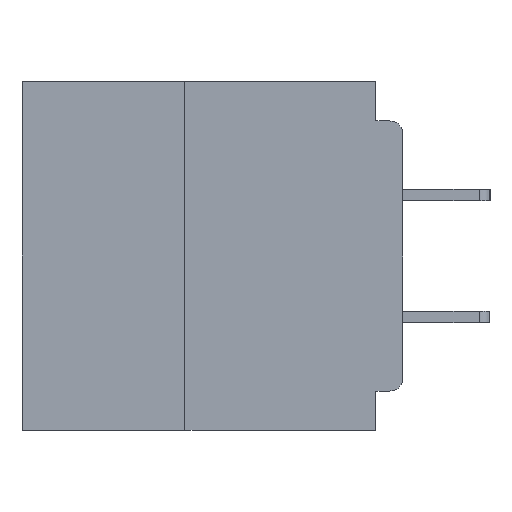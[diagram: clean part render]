
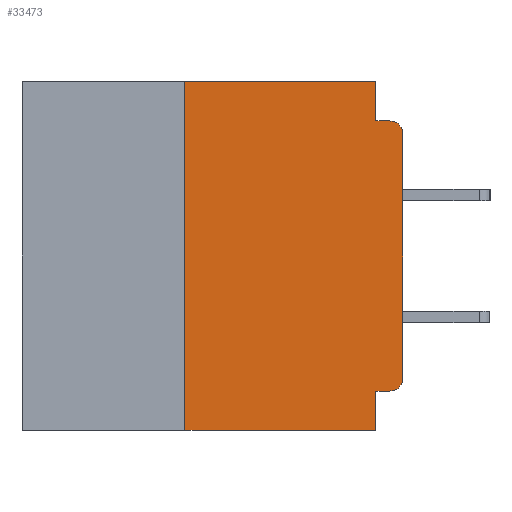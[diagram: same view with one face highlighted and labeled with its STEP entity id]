
A CAD part, left-side view. The second image highlights one B-rep face of the part: STEP entity #33473.
In plain terms, the highlighted planar face has unit normal (-1, 0, 0).
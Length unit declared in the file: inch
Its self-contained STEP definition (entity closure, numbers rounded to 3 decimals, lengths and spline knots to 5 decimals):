
#336 = LINE ( 'NONE', #9048, #36361 ) ;
#529 = LINE ( 'NONE', #7827, #14073 ) ;
#898 = EDGE_CURVE ( 'NONE', #4974, #16801, #36397, .T. ) ;
#1073 = EDGE_CURVE ( 'NONE', #11123, #27617, #28911, .T. ) ;
#1193 = EDGE_CURVE ( 'NONE', #33816, #10783, #336, .T. ) ;
#1250 = EDGE_CURVE ( 'NONE', #16801, #27617, #6198, .T. ) ;
#1259 = CARTESIAN_POINT ( 'NONE',  ( 0., 0.031, 0. ) ) ;
#1301 = EDGE_CURVE ( 'NONE', #33816, #4974, #20012, .T. ) ;
#1632 = ORIENTED_EDGE ( 'NONE', *, *, #10062, .T. ) ;
#2718 = CARTESIAN_POINT ( 'NONE',  ( 0., 0.031, -0.4 ) ) ;
#4177 = VECTOR ( 'NONE', #7340, 39.37008 ) ;
#4974 = VERTEX_POINT ( 'NONE', #30198 ) ;
#5546 = ORIENTED_EDGE ( 'NONE', *, *, #9873, .F. ) ;
#6198 = CIRCLE ( 'NONE', #20914, 0.015 ) ;
#7340 = DIRECTION ( 'NONE',  ( 0., 0., -1. ) ) ;
#7827 = CARTESIAN_POINT ( 'NONE',  ( 0., 0.25, -0.4 ) ) ;
#8604 = VECTOR ( 'NONE', #20373, 39.37008 ) ;
#9048 = CARTESIAN_POINT ( 'NONE',  ( 0., 0., -0.355 ) ) ;
#9590 = CARTESIAN_POINT ( 'NONE',  ( 0., 0., -0.045 ) ) ;
#9873 = EDGE_CURVE ( 'NONE', #22394, #11123, #27360, .T. ) ;
#9991 = EDGE_CURVE ( 'NONE', #13685, #15500, #529, .T. ) ;
#10062 = EDGE_CURVE ( 'NONE', #13685, #33516, #19256, .T. ) ;
#10125 = EDGE_CURVE ( 'NONE', #10783, #33516, #16416, .T. ) ;
#10783 = VERTEX_POINT ( 'NONE', #28747 ) ;
#11123 = VERTEX_POINT ( 'NONE', #24500 ) ;
#12314 = ORIENTED_EDGE ( 'NONE', *, *, #898, .T. ) ;
#13685 = VERTEX_POINT ( 'NONE', #15130 ) ;
#13720 = CARTESIAN_POINT ( 'NONE',  ( 0., 0.437, 0. ) ) ;
#13733 = CARTESIAN_POINT ( 'NONE',  ( 0., 0., 0. ) ) ;
#13835 = CARTESIAN_POINT ( 'NONE',  ( 0., 0.015, -0.355 ) ) ;
#14073 = VECTOR ( 'NONE', #16563, 39.37008 ) ;
#14253 = DIRECTION ( 'NONE',  ( 0., 1., 0. ) ) ;
#14795 = CARTESIAN_POINT ( 'NONE',  ( 0., 0.015, -0.045 ) ) ;
#15130 = CARTESIAN_POINT ( 'NONE',  ( 0., 0.25, -0.4 ) ) ;
#15298 = DIRECTION ( 'NONE',  ( 1., 0., 0. ) ) ;
#15500 = VERTEX_POINT ( 'NONE', #15547 ) ;
#15547 = CARTESIAN_POINT ( 'NONE',  ( 0., 0.25, 0. ) ) ;
#16416 = LINE ( 'NONE', #2718, #8604 ) ;
#16563 = DIRECTION ( 'NONE',  ( 0., 0., 1. ) ) ;
#16748 = CARTESIAN_POINT ( 'NONE',  ( 0., 0., -0.06 ) ) ;
#16801 = VERTEX_POINT ( 'NONE', #16748 ) ;
#16952 = CARTESIAN_POINT ( 'NONE',  ( 0., 0.437, -0.4 ) ) ;
#17098 = ORIENTED_EDGE ( 'NONE', *, *, #10125, .F. ) ;
#18215 = CARTESIAN_POINT ( 'NONE',  ( 0., 0.437, 0. ) ) ;
#18489 = CARTESIAN_POINT ( 'NONE',  ( 0., 0.031, -0.4 ) ) ;
#19256 = LINE ( 'NONE', #16952, #26035 ) ;
#19557 = CARTESIAN_POINT ( 'NONE',  ( 0., 0.015, -0.06 ) ) ;
#19602 = DIRECTION ( 'NONE',  ( 0., 0., 1. ) ) ;
#20012 = CIRCLE ( 'NONE', #30288, 0.015 ) ;
#20302 = ORIENTED_EDGE ( 'NONE', *, *, #1301, .T. ) ;
#20373 = DIRECTION ( 'NONE',  ( 0., 0., -1. ) ) ;
#20914 = AXIS2_PLACEMENT_3D ( 'NONE', #19557, #22013, #32410 ) ;
#21160 = FACE_OUTER_BOUND ( 'NONE', #21373, .T. ) ;
#21373 = EDGE_LOOP ( 'NONE', ( #12314, #27791, #36396, #5546, #30814, #26051, #1632, #17098, #22556, #20302 ) ) ;
#21990 = VECTOR ( 'NONE', #19602, 39.37008 ) ;
#22013 = DIRECTION ( 'NONE',  ( -1., 0., 0. ) ) ;
#22394 = VERTEX_POINT ( 'NONE', #1259 ) ;
#22556 = ORIENTED_EDGE ( 'NONE', *, *, #1193, .F. ) ;
#22949 = DIRECTION ( 'NONE',  ( 0., -1., 0. ) ) ;
#24500 = CARTESIAN_POINT ( 'NONE',  ( 0., 0.031, -0.045 ) ) ;
#24629 = VECTOR ( 'NONE', #36386, 39.37008 ) ;
#26035 = VECTOR ( 'NONE', #22949, 39.37008 ) ;
#26051 = ORIENTED_EDGE ( 'NONE', *, *, #9991, .F. ) ;
#26084 = CARTESIAN_POINT ( 'NONE',  ( 0., 0.015, -0.34 ) ) ;
#27120 = DIRECTION ( 'NONE',  ( 0., 0., -1. ) ) ;
#27195 = DIRECTION ( 'NONE',  ( -1., 0., 0. ) ) ;
#27360 = LINE ( 'NONE', #27711, #4177 ) ;
#27617 = VERTEX_POINT ( 'NONE', #14795 ) ;
#27711 = CARTESIAN_POINT ( 'NONE',  ( 0., 0.031, 0. ) ) ;
#27791 = ORIENTED_EDGE ( 'NONE', *, *, #1250, .T. ) ;
#28747 = CARTESIAN_POINT ( 'NONE',  ( 0., 0.031, -0.355 ) ) ;
#28911 = LINE ( 'NONE', #9590, #35156 ) ;
#29474 = AXIS2_PLACEMENT_3D ( 'NONE', #18215, #15298, #35030 ) ;
#30198 = CARTESIAN_POINT ( 'NONE',  ( 0., 0., -0.34 ) ) ;
#30288 = AXIS2_PLACEMENT_3D ( 'NONE', #26084, #27195, #27120 ) ;
#30814 = ORIENTED_EDGE ( 'NONE', *, *, #35582, .F. ) ;
#31890 = LINE ( 'NONE', #13720, #24629 ) ;
#32290 = DIRECTION ( 'NONE',  ( 0., -1., 0. ) ) ;
#32382 = PLANE ( 'NONE',  #29474 ) ;
#32410 = DIRECTION ( 'NONE',  ( 0., 0., -1. ) ) ;
#33473 = ADVANCED_FACE ( 'NONE', ( #21160 ), #32382, .F. ) ;
#33516 = VERTEX_POINT ( 'NONE', #18489 ) ;
#33816 = VERTEX_POINT ( 'NONE', #13835 ) ;
#35030 = DIRECTION ( 'NONE',  ( 0., 0., -1. ) ) ;
#35156 = VECTOR ( 'NONE', #32290, 39.37008 ) ;
#35582 = EDGE_CURVE ( 'NONE', #15500, #22394, #31890, .T. ) ;
#36361 = VECTOR ( 'NONE', #14253, 39.37008 ) ;
#36386 = DIRECTION ( 'NONE',  ( 0., -1., 0. ) ) ;
#36396 = ORIENTED_EDGE ( 'NONE', *, *, #1073, .F. ) ;
#36397 = LINE ( 'NONE', #13733, #21990 ) ;
